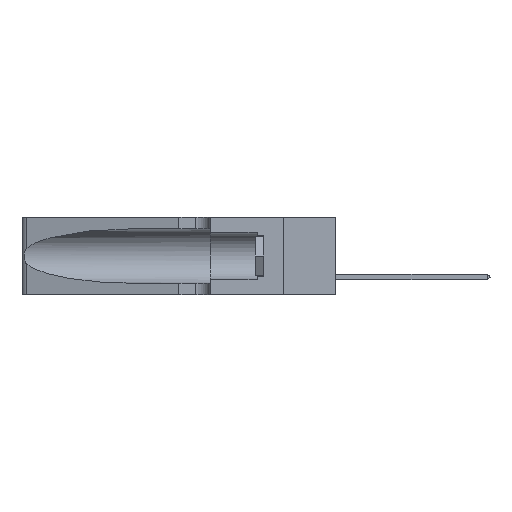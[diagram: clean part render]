
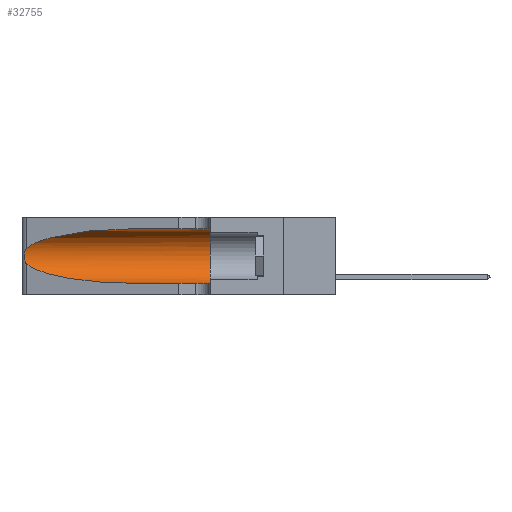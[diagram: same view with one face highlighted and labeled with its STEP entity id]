
A CAD part, left-side view. The second image highlights one B-rep face of the part: STEP entity #32755.
In plain terms, the highlighted cylindrical face has radius 3.308 mm (diameter 6.617 mm), a partial arc.
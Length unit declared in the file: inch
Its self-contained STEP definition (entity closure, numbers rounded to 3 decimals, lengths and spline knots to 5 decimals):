
#229 =( BOUNDED_CURVE ( )  B_SPLINE_CURVE ( 3, ( #22579, #33422, #31007, #25869 ),
 .UNSPECIFIED., .F., .T. ) 
 B_SPLINE_CURVE_WITH_KNOTS ( ( 4, 4 ),
 ( 1.5708, 2.84003 ),
 .UNSPECIFIED. ) 
 CURVE ( )  GEOMETRIC_REPRESENTATION_ITEM ( )  RATIONAL_B_SPLINE_CURVE ( ( 1., 0.87, 0.87, 1. ) ) 
 REPRESENTATION_ITEM ( '' )  );
#256 = LINE ( 'NONE', #22186, #26363 ) ;
#620 = EDGE_CURVE ( 'NONE', #5308, #31043, #21553, .T. ) ;
#1372 = DIRECTION ( 'NONE',  ( 0., 0., 1. ) ) ;
#2166 = CYLINDRICAL_SURFACE ( 'NONE', #29968, 0.13025 ) ;
#2491 = EDGE_CURVE ( 'NONE', #31043, #19769, #7859, .T. ) ;
#2906 = CARTESIAN_POINT ( 'NONE',  ( 0.1305, 0.72297, 0.05475 ) ) ;
#3776 = CARTESIAN_POINT ( 'NONE',  ( 0.1305, 1.61858, 0.185 ) ) ;
#4886 = B_SPLINE_CURVE_WITH_KNOTS ( 'NONE', 3,
 ( #22312, #23326, #7704, #14194, #28504, #31146, #26895, #8208, #29168, #26432, #18781, #8553, #21412, #22340 ),
 .UNSPECIFIED., .F., .F.,
 ( 4, 2, 2, 2, 2, 2, 4 ),
 ( 0., 0.00027, 0.00053, 0.00107, 0.0016, 0.00187, 0.00214 ),
 .UNSPECIFIED. ) ;
#5308 = VERTEX_POINT ( 'NONE', #11678 ) ;
#5585 = CARTESIAN_POINT ( 'NONE',  ( 0.1305, 0.35, 0.05475 ) ) ;
#5814 = CARTESIAN_POINT ( 'NONE',  ( 0.1305, 0.72297, 0.31525 ) ) ;
#6338 = ORIENTED_EDGE ( 'NONE', *, *, #24686, .F. ) ;
#7061 = CIRCLE ( 'NONE', #8084, 0.13025 ) ;
#7367 = CARTESIAN_POINT ( 'NONE',  ( 0.1305, 1.61858, 0.05475 ) ) ;
#7704 = CARTESIAN_POINT ( 'NONE',  ( 0.25639, 1.23184, 0.21858 ) ) ;
#7859 = LINE ( 'NONE', #7367, #12335 ) ;
#7941 = VERTEX_POINT ( 'NONE', #25533 ) ;
#8084 = AXIS2_PLACEMENT_3D ( 'NONE', #19682, #9430, #1372 ) ;
#8208 = CARTESIAN_POINT ( 'NONE',  ( 0.26075, 1.23896, 0.178 ) ) ;
#8553 = CARTESIAN_POINT ( 'NONE',  ( 0.25639, 1.23186, 0.15144 ) ) ;
#9430 = DIRECTION ( 'NONE',  ( 0., 1., 0. ) ) ;
#9908 = FACE_OUTER_BOUND ( 'NONE', #15382, .T. ) ;
#10307 = ORIENTED_EDGE ( 'NONE', *, *, #27489, .F. ) ;
#10846 = CARTESIAN_POINT ( 'NONE',  ( 0.25487, 1.22718, 0.14631 ) ) ;
#11678 = CARTESIAN_POINT ( 'NONE',  ( 0.25487, 1.22718, 0.14631 ) ) ;
#12335 = VECTOR ( 'NONE', #27857, 39.37008 ) ;
#14194 = CARTESIAN_POINT ( 'NONE',  ( 0.25787, 1.23484, 0.2124 ) ) ;
#15107 = VERTEX_POINT ( 'NONE', #22094 ) ;
#15382 = EDGE_LOOP ( 'NONE', ( #16651, #23049, #28581, #24876, #6338, #10307 ) ) ;
#16651 = ORIENTED_EDGE ( 'NONE', *, *, #28319, .T. ) ;
#18781 = CARTESIAN_POINT ( 'NONE',  ( 0.25789, 1.23486, 0.15765 ) ) ;
#19682 = CARTESIAN_POINT ( 'NONE',  ( 0.1305, 0.35, 0.185 ) ) ;
#19769 = VERTEX_POINT ( 'NONE', #5585 ) ;
#21412 = CARTESIAN_POINT ( 'NONE',  ( 0.25555, 1.22993, 0.14849 ) ) ;
#21553 =( BOUNDED_CURVE ( )  B_SPLINE_CURVE ( 3, ( #10846, #24011, #26343, #28957 ),
 .UNSPECIFIED., .F., .F. ) 
 B_SPLINE_CURVE_WITH_KNOTS ( ( 4, 4 ),
 ( 3.44316, 4.71239 ),
 .UNSPECIFIED. ) 
 CURVE ( )  GEOMETRIC_REPRESENTATION_ITEM ( )  RATIONAL_B_SPLINE_CURVE ( ( 1., 0.87, 0.87, 1. ) ) 
 REPRESENTATION_ITEM ( '' )  );
#22006 = DIRECTION ( 'NONE',  ( 0., -1., 0. ) ) ;
#22094 = CARTESIAN_POINT ( 'NONE',  ( 0.1305, 0.35, 0.31525 ) ) ;
#22186 = CARTESIAN_POINT ( 'NONE',  ( 0.1305, 1.61858, 0.31525 ) ) ;
#22312 = CARTESIAN_POINT ( 'NONE',  ( 0.25487, 1.22718, 0.22369 ) ) ;
#22340 = CARTESIAN_POINT ( 'NONE',  ( 0.25487, 1.22718, 0.14631 ) ) ;
#22579 = CARTESIAN_POINT ( 'NONE',  ( 0.1305, 0.72297, 0.31525 ) ) ;
#22971 = DIRECTION ( 'NONE',  ( 0., -1., 0. ) ) ;
#23049 = ORIENTED_EDGE ( 'NONE', *, *, #32634, .T. ) ;
#23326 = CARTESIAN_POINT ( 'NONE',  ( 0.25555, 1.22994, 0.2215 ) ) ;
#24011 = CARTESIAN_POINT ( 'NONE',  ( 0.2373, 1.15595, 0.08982 ) ) ;
#24686 = EDGE_CURVE ( 'NONE', #15107, #19769, #7061, .T. ) ;
#24876 = ORIENTED_EDGE ( 'NONE', *, *, #2491, .T. ) ;
#25533 = CARTESIAN_POINT ( 'NONE',  ( 0.25487, 1.22718, 0.22369 ) ) ;
#25869 = CARTESIAN_POINT ( 'NONE',  ( 0.25487, 1.22718, 0.22369 ) ) ;
#26343 = CARTESIAN_POINT ( 'NONE',  ( 0.18966, 0.96281, 0.05475 ) ) ;
#26363 = VECTOR ( 'NONE', #22971, 39.37008 ) ;
#26432 = CARTESIAN_POINT ( 'NONE',  ( 0.25856, 1.23593, 0.16098 ) ) ;
#26895 = CARTESIAN_POINT ( 'NONE',  ( 0.26075, 1.23896, 0.19203 ) ) ;
#27235 = DIRECTION ( 'NONE',  ( 0., 0., -1. ) ) ;
#27489 = EDGE_CURVE ( 'NONE', #30788, #15107, #256, .T. ) ;
#27857 = DIRECTION ( 'NONE',  ( 0., -1., 0. ) ) ;
#28319 = EDGE_CURVE ( 'NONE', #30788, #7941, #229, .T. ) ;
#28504 = CARTESIAN_POINT ( 'NONE',  ( 0.25854, 1.2359, 0.20912 ) ) ;
#28581 = ORIENTED_EDGE ( 'NONE', *, *, #620, .T. ) ;
#28957 = CARTESIAN_POINT ( 'NONE',  ( 0.1305, 0.72297, 0.05475 ) ) ;
#29168 = CARTESIAN_POINT ( 'NONE',  ( 0.26017, 1.23833, 0.17102 ) ) ;
#29968 = AXIS2_PLACEMENT_3D ( 'NONE', #3776, #22006, #27235 ) ;
#30788 = VERTEX_POINT ( 'NONE', #5814 ) ;
#31007 = CARTESIAN_POINT ( 'NONE',  ( 0.2373, 1.15595, 0.28018 ) ) ;
#31043 = VERTEX_POINT ( 'NONE', #2906 ) ;
#31146 = CARTESIAN_POINT ( 'NONE',  ( 0.26018, 1.23835, 0.19895 ) ) ;
#32634 = EDGE_CURVE ( 'NONE', #7941, #5308, #4886, .T. ) ;
#32755 = ADVANCED_FACE ( 'NONE', ( #9908 ), #2166, .F. ) ;
#33422 = CARTESIAN_POINT ( 'NONE',  ( 0.18966, 0.96281, 0.31525 ) ) ;
